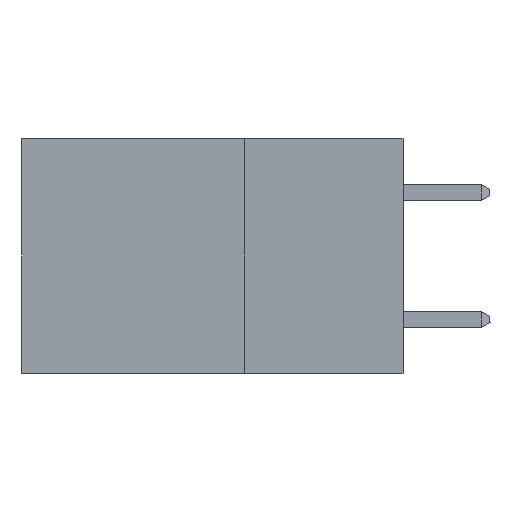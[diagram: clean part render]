
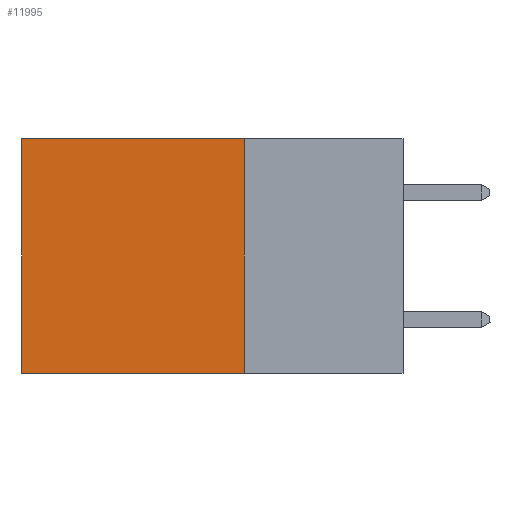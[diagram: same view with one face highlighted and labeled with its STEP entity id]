
A CAD part, left-side view. The second image highlights one B-rep face of the part: STEP entity #11995.
In plain terms, the highlighted planar face has unit normal (-1, 0, 0).
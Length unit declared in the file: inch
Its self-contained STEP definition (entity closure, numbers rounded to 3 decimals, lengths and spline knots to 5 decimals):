
#1314 = VERTEX_POINT ( 'NONE', #3186 ) ;
#1448 = VERTEX_POINT ( 'NONE', #11915 ) ;
#1572 = PLANE ( 'NONE',  #9926 ) ;
#1641 = CARTESIAN_POINT ( 'NONE',  ( 0.2875, 0.25, 0. ) ) ;
#3186 = CARTESIAN_POINT ( 'NONE',  ( 0.2875, 0.25, -0.37 ) ) ;
#3252 = ORIENTED_EDGE ( 'NONE', *, *, #11836, .F. ) ;
#3416 = DIRECTION ( 'NONE',  ( 0., 0., -1. ) ) ;
#3574 = CARTESIAN_POINT ( 'NONE',  ( 0.2875, 0.25, 0. ) ) ;
#4464 = EDGE_CURVE ( 'NONE', #13734, #9309, #10464, .T. ) ;
#4497 = VECTOR ( 'NONE', #15680, 39.37008 ) ;
#4612 = ORIENTED_EDGE ( 'NONE', *, *, #7088, .F. ) ;
#5154 = LINE ( 'NONE', #12603, #13242 ) ;
#5858 = FACE_OUTER_BOUND ( 'NONE', #19441, .T. ) ;
#7088 = EDGE_CURVE ( 'NONE', #1314, #1448, #5154, .T. ) ;
#8556 = CARTESIAN_POINT ( 'NONE',  ( 0.2875, 0.25, 0. ) ) ;
#9309 = VERTEX_POINT ( 'NONE', #17027 ) ;
#9485 = CARTESIAN_POINT ( 'NONE',  ( 0.2875, 0.6, 0. ) ) ;
#9512 = DIRECTION ( 'NONE',  ( 0., 1., 0. ) ) ;
#9926 = AXIS2_PLACEMENT_3D ( 'NONE', #1641, #13765, #3416 ) ;
#10464 = LINE ( 'NONE', #19886, #18600 ) ;
#11243 = DIRECTION ( 'NONE',  ( 0., 0., -1. ) ) ;
#11836 = EDGE_CURVE ( 'NONE', #13734, #1314, #22295, .T. ) ;
#11915 = CARTESIAN_POINT ( 'NONE',  ( 0.2875, 0.6, -0.37 ) ) ;
#11995 = ADVANCED_FACE ( 'NONE', ( #5858 ), #1572, .F. ) ;
#12501 = ORIENTED_EDGE ( 'NONE', *, *, #4464, .T. ) ;
#12603 = CARTESIAN_POINT ( 'NONE',  ( 0.2875, 0.25, -0.37 ) ) ;
#13242 = VECTOR ( 'NONE', #16158, 39.37008 ) ;
#13734 = VERTEX_POINT ( 'NONE', #8556 ) ;
#13765 = DIRECTION ( 'NONE',  ( 1., 0., 0. ) ) ;
#15680 = DIRECTION ( 'NONE',  ( 0., 0., -1. ) ) ;
#16158 = DIRECTION ( 'NONE',  ( 0., 1., 0. ) ) ;
#17027 = CARTESIAN_POINT ( 'NONE',  ( 0.2875, 0.6, 0. ) ) ;
#18600 = VECTOR ( 'NONE', #9512, 39.37008 ) ;
#19441 = EDGE_LOOP ( 'NONE', ( #21887, #4612, #3252, #12501 ) ) ;
#19886 = CARTESIAN_POINT ( 'NONE',  ( 0.2875, 0.25, 0. ) ) ;
#20558 = LINE ( 'NONE', #9485, #21067 ) ;
#20773 = EDGE_CURVE ( 'NONE', #9309, #1448, #20558, .T. ) ;
#21067 = VECTOR ( 'NONE', #11243, 39.37008 ) ;
#21887 = ORIENTED_EDGE ( 'NONE', *, *, #20773, .T. ) ;
#22295 = LINE ( 'NONE', #3574, #4497 ) ;
